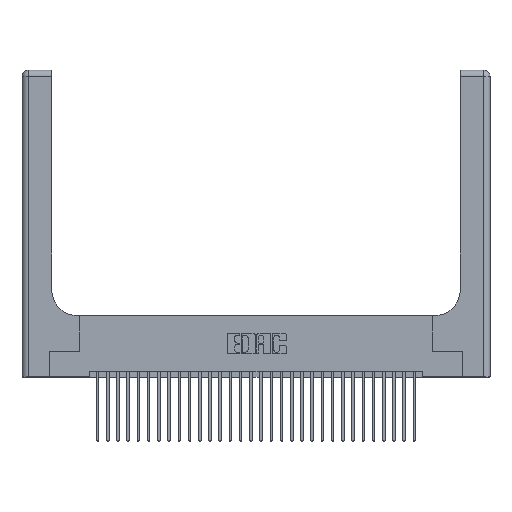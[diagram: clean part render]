
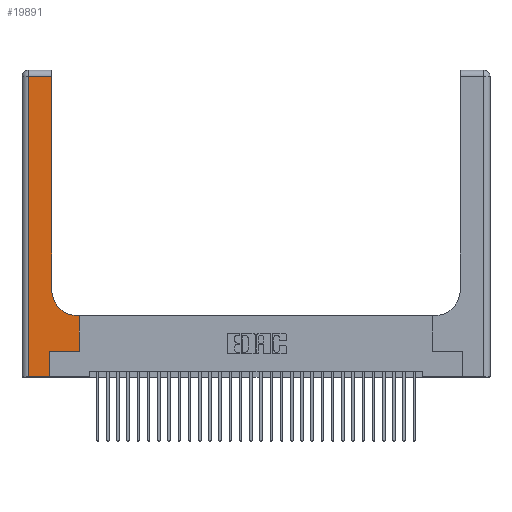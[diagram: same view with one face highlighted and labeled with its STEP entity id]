
A CAD part, top view. The second image highlights one B-rep face of the part: STEP entity #19891.
In plain terms, the highlighted planar face has unit normal (0, 0, 1).
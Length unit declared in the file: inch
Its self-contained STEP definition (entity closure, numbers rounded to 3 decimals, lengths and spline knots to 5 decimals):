
#294 = LINE ( 'NONE', #15838, #25568 ) ;
#382 = VERTEX_POINT ( 'NONE', #5924 ) ;
#881 = VECTOR ( 'NONE', #23953, 39.37008 ) ;
#972 = DIRECTION ( 'NONE',  ( 1., 0., 0. ) ) ;
#1248 = VERTEX_POINT ( 'NONE', #23636 ) ;
#1917 = CARTESIAN_POINT ( 'NONE',  ( 0.2915, 3., 0.37 ) ) ;
#2798 = ORIENTED_EDGE ( 'NONE', *, *, #30296, .T. ) ;
#3340 = CARTESIAN_POINT ( 'NONE',  ( 0., 3., 0.37 ) ) ;
#3741 = ORIENTED_EDGE ( 'NONE', *, *, #7161, .T. ) ;
#4387 = EDGE_CURVE ( 'NONE', #1248, #11885, #31242, .T. ) ;
#4463 = CIRCLE ( 'NONE', #5123, 0.25 ) ;
#4732 = VERTEX_POINT ( 'NONE', #25167 ) ;
#5057 = LINE ( 'NONE', #30106, #10798 ) ;
#5123 = AXIS2_PLACEMENT_3D ( 'NONE', #30270, #15605, #972 ) ;
#5924 = CARTESIAN_POINT ( 'NONE',  ( 0.2915, 2.94, 0.37 ) ) ;
#6436 = CARTESIAN_POINT ( 'NONE',  ( 0.5585, 0.25, 0.37 ) ) ;
#6585 = VERTEX_POINT ( 'NONE', #25000 ) ;
#7161 = EDGE_CURVE ( 'NONE', #17319, #1248, #5057, .T. ) ;
#7245 = VERTEX_POINT ( 'NONE', #18115 ) ;
#7246 = ORIENTED_EDGE ( 'NONE', *, *, #13338, .T. ) ;
#7674 = DIRECTION ( 'NONE',  ( 0., -1., 0. ) ) ;
#8142 = LINE ( 'NONE', #1917, #881 ) ;
#8226 = EDGE_LOOP ( 'NONE', ( #27377, #2798, #16742, #7246, #16003, #9703, #3741, #18871, #12920 ) ) ;
#8251 = PLANE ( 'NONE',  #18379 ) ;
#9037 = DIRECTION ( 'NONE',  ( -1., 0., 0. ) ) ;
#9158 = VECTOR ( 'NONE', #7674, 39.37008 ) ;
#9703 = ORIENTED_EDGE ( 'NONE', *, *, #31341, .T. ) ;
#10523 = DIRECTION ( 'NONE',  ( 0., 1., 0. ) ) ;
#10610 = LINE ( 'NONE', #20152, #30889 ) ;
#10709 = DIRECTION ( 'NONE',  ( -1., 0., 0. ) ) ;
#10798 = VECTOR ( 'NONE', #10523, 39.37008 ) ;
#10883 = DIRECTION ( 'NONE',  ( 1., 0., 0. ) ) ;
#10921 = CARTESIAN_POINT ( 'NONE',  ( 0., 0., 0.37 ) ) ;
#11337 = EDGE_CURVE ( 'NONE', #11885, #4732, #4463, .T. ) ;
#11885 = VERTEX_POINT ( 'NONE', #27349 ) ;
#12212 = CARTESIAN_POINT ( 'NONE',  ( 0.06, 0., 0.37 ) ) ;
#12920 = ORIENTED_EDGE ( 'NONE', *, *, #11337, .T. ) ;
#13338 = EDGE_CURVE ( 'NONE', #14630, #6585, #20802, .T. ) ;
#13554 = EDGE_CURVE ( 'NONE', #4732, #382, #8142, .T. ) ;
#14362 = VECTOR ( 'NONE', #10883, 39.37008 ) ;
#14630 = VERTEX_POINT ( 'NONE', #12212 ) ;
#15605 = DIRECTION ( 'NONE',  ( 0., 0., -1. ) ) ;
#15838 = CARTESIAN_POINT ( 'NONE',  ( 0.269, 0., 0.37 ) ) ;
#16003 = ORIENTED_EDGE ( 'NONE', *, *, #22565, .T. ) ;
#16146 = CARTESIAN_POINT ( 'NONE',  ( 0.06, 2.94, 0.37 ) ) ;
#16742 = ORIENTED_EDGE ( 'NONE', *, *, #26645, .T. ) ;
#17319 = VERTEX_POINT ( 'NONE', #6436 ) ;
#18115 = CARTESIAN_POINT ( 'NONE',  ( 0.269, 0.25, 0.37 ) ) ;
#18379 = AXIS2_PLACEMENT_3D ( 'NONE', #3340, #25373, #10709 ) ;
#18871 = ORIENTED_EDGE ( 'NONE', *, *, #4387, .T. ) ;
#19891 = ADVANCED_FACE ( 'NONE', ( #19927 ), #8251, .F. ) ;
#19927 = FACE_OUTER_BOUND ( 'NONE', #8226, .T. ) ;
#20020 = VECTOR ( 'NONE', #30485, 39.37008 ) ;
#20152 = CARTESIAN_POINT ( 'NONE',  ( 0., 2.94, 0.37 ) ) ;
#20802 = LINE ( 'NONE', #10921, #20020 ) ;
#20869 = LINE ( 'NONE', #25539, #14362 ) ;
#22331 = CARTESIAN_POINT ( 'NONE',  ( 0.06, 3., 0.37 ) ) ;
#22565 = EDGE_CURVE ( 'NONE', #6585, #7245, #294, .T. ) ;
#22622 = DIRECTION ( 'NONE',  ( -1., 0., 0. ) ) ;
#23220 = VECTOR ( 'NONE', #9037, 39.37008 ) ;
#23232 = DIRECTION ( 'NONE',  ( 0., 1., 0. ) ) ;
#23636 = CARTESIAN_POINT ( 'NONE',  ( 0.5585, 0.6, 0.37 ) ) ;
#23953 = DIRECTION ( 'NONE',  ( 0., 1., 0. ) ) ;
#24555 = VERTEX_POINT ( 'NONE', #16146 ) ;
#25000 = CARTESIAN_POINT ( 'NONE',  ( 0.269, 0., 0.37 ) ) ;
#25167 = CARTESIAN_POINT ( 'NONE',  ( 0.2915, 0.85, 0.37 ) ) ;
#25373 = DIRECTION ( 'NONE',  ( 0., 0., -1. ) ) ;
#25539 = CARTESIAN_POINT ( 'NONE',  ( 0.269, 0.25, 0.37 ) ) ;
#25568 = VECTOR ( 'NONE', #23232, 39.37008 ) ;
#26164 = CARTESIAN_POINT ( 'NONE',  ( 0.2915, 0.6, 0.37 ) ) ;
#26645 = EDGE_CURVE ( 'NONE', #24555, #14630, #28686, .T. ) ;
#27349 = CARTESIAN_POINT ( 'NONE',  ( 0.5415, 0.6, 0.37 ) ) ;
#27377 = ORIENTED_EDGE ( 'NONE', *, *, #13554, .T. ) ;
#28686 = LINE ( 'NONE', #22331, #9158 ) ;
#30106 = CARTESIAN_POINT ( 'NONE',  ( 0.5585, 0.25, 0.37 ) ) ;
#30270 = CARTESIAN_POINT ( 'NONE',  ( 0.5415, 0.85, 0.37 ) ) ;
#30296 = EDGE_CURVE ( 'NONE', #382, #24555, #10610, .T. ) ;
#30485 = DIRECTION ( 'NONE',  ( 1., 0., 0. ) ) ;
#30889 = VECTOR ( 'NONE', #22622, 39.37008 ) ;
#31242 = LINE ( 'NONE', #26164, #23220 ) ;
#31341 = EDGE_CURVE ( 'NONE', #7245, #17319, #20869, .T. ) ;
